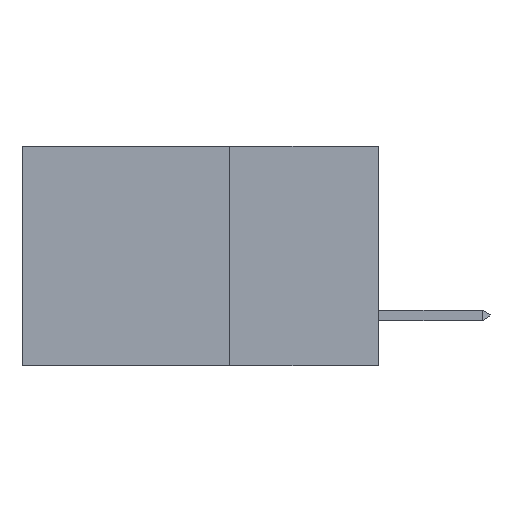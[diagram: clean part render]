
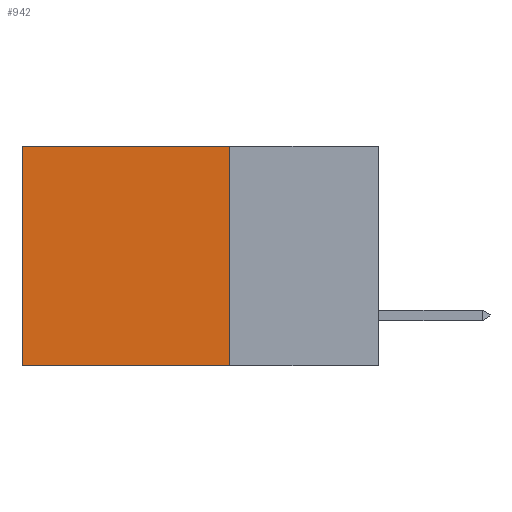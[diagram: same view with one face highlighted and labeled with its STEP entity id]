
A CAD part, left-side view. The second image highlights one B-rep face of the part: STEP entity #942.
In plain terms, the highlighted planar face has unit normal (-1, 0, 0).
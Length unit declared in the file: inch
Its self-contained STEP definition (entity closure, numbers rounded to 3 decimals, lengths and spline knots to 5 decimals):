
#766 = ORIENTED_EDGE ( 'NONE', *, *, #5603, .F. ) ;
#942 = ADVANCED_FACE ( 'NONE', ( #12572 ), #7533, .F. ) ;
#1698 = VECTOR ( 'NONE', #11904, 39.37008 ) ;
#1861 = ORIENTED_EDGE ( 'NONE', *, *, #8580, .T. ) ;
#1892 = VERTEX_POINT ( 'NONE', #6721 ) ;
#2133 = CARTESIAN_POINT ( 'NONE',  ( 0.2615, 0.25, 0. ) ) ;
#2502 = VECTOR ( 'NONE', #7589, 39.37008 ) ;
#2831 = CARTESIAN_POINT ( 'NONE',  ( 0.2615, 0.25, -0.37 ) ) ;
#3101 = LINE ( 'NONE', #4996, #6039 ) ;
#3172 = VERTEX_POINT ( 'NONE', #7400 ) ;
#3379 = LINE ( 'NONE', #11277, #2502 ) ;
#4201 = LINE ( 'NONE', #2133, #1698 ) ;
#4996 = CARTESIAN_POINT ( 'NONE',  ( 0.2615, 0.6, -0.37 ) ) ;
#5213 = EDGE_LOOP ( 'NONE', ( #1861, #8368, #766, #12773 ) ) ;
#5603 = EDGE_CURVE ( 'NONE', #8294, #7197, #3379, .T. ) ;
#6039 = VECTOR ( 'NONE', #7064, 39.37008 ) ;
#6424 = CARTESIAN_POINT ( 'NONE',  ( 0.2615, 0.25, 0. ) ) ;
#6430 = CARTESIAN_POINT ( 'NONE',  ( 0.2615, 0.25, -0.37 ) ) ;
#6695 = DIRECTION ( 'NONE',  ( 0., 0., -1. ) ) ;
#6721 = CARTESIAN_POINT ( 'NONE',  ( 0.2615, 0.6, 0. ) ) ;
#7064 = DIRECTION ( 'NONE',  ( 0., 0., -1. ) ) ;
#7197 = VERTEX_POINT ( 'NONE', #9007 ) ;
#7400 = CARTESIAN_POINT ( 'NONE',  ( 0.2615, 0.6, -0.37 ) ) ;
#7533 = PLANE ( 'NONE',  #11017 ) ;
#7589 = DIRECTION ( 'NONE',  ( 0., 0., -1. ) ) ;
#8294 = VERTEX_POINT ( 'NONE', #6424 ) ;
#8368 = ORIENTED_EDGE ( 'NONE', *, *, #11021, .F. ) ;
#8580 = EDGE_CURVE ( 'NONE', #1892, #3172, #3101, .T. ) ;
#9007 = CARTESIAN_POINT ( 'NONE',  ( 0.2615, 0.25, -0.37 ) ) ;
#9306 = LINE ( 'NONE', #2831, #11779 ) ;
#9313 = EDGE_CURVE ( 'NONE', #8294, #1892, #4201, .T. ) ;
#11017 = AXIS2_PLACEMENT_3D ( 'NONE', #6430, #12519, #6695 ) ;
#11021 = EDGE_CURVE ( 'NONE', #7197, #3172, #9306, .T. ) ;
#11277 = CARTESIAN_POINT ( 'NONE',  ( 0.2615, 0.25, -0.37 ) ) ;
#11779 = VECTOR ( 'NONE', #11780, 39.37008 ) ;
#11780 = DIRECTION ( 'NONE',  ( 0., 1., 0. ) ) ;
#11904 = DIRECTION ( 'NONE',  ( 0., 1., 0. ) ) ;
#12519 = DIRECTION ( 'NONE',  ( 1., 0., 0. ) ) ;
#12572 = FACE_OUTER_BOUND ( 'NONE', #5213, .T. ) ;
#12773 = ORIENTED_EDGE ( 'NONE', *, *, #9313, .T. ) ;
